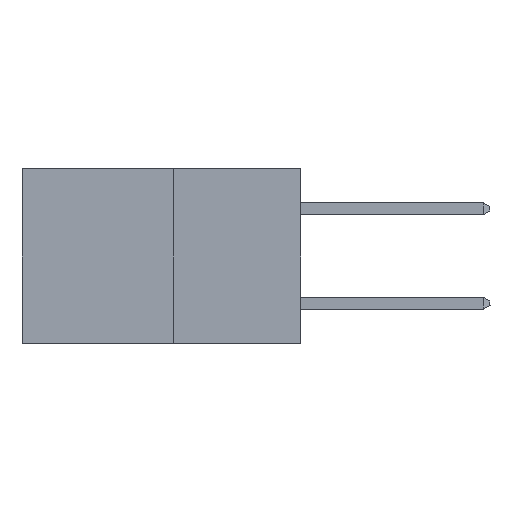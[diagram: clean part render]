
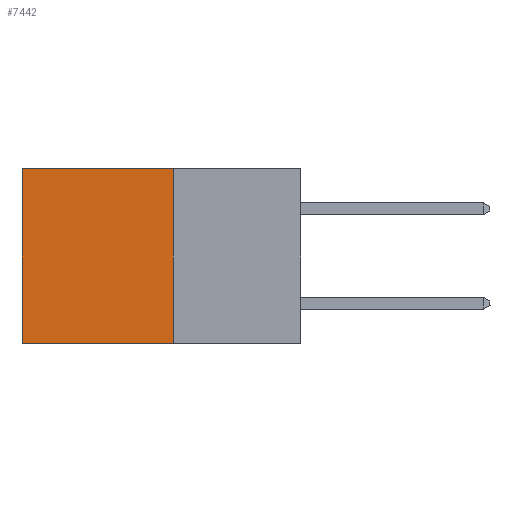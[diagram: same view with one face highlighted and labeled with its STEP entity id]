
A CAD part, left-side view. The second image highlights one B-rep face of the part: STEP entity #7442.
In plain terms, the highlighted planar face has unit normal (-1, 0, 0).
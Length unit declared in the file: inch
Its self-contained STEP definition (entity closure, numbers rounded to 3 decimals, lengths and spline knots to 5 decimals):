
#1515 = EDGE_LOOP ( 'NONE', ( #19555, #17961, #22733, #8371 ) ) ;
#1623 = LINE ( 'NONE', #22899, #10051 ) ;
#2425 = LINE ( 'NONE', #10143, #11977 ) ;
#2489 = VERTEX_POINT ( 'NONE', #14264 ) ;
#5744 = VERTEX_POINT ( 'NONE', #11250 ) ;
#7442 = ADVANCED_FACE ( 'NONE', ( #20026 ), #17059, .F. ) ;
#7711 = EDGE_CURVE ( 'NONE', #5744, #18643, #14528, .T. ) ;
#7771 = DIRECTION ( 'NONE',  ( 0., 0., -1. ) ) ;
#8371 = ORIENTED_EDGE ( 'NONE', *, *, #14161, .T. ) ;
#10039 = DIRECTION ( 'NONE',  ( 1., 0., 0. ) ) ;
#10051 = VECTOR ( 'NONE', #12383, 39.37008 ) ;
#10143 = CARTESIAN_POINT ( 'NONE',  ( 0.277, 0.27, -0.37 ) ) ;
#11250 = CARTESIAN_POINT ( 'NONE',  ( 0.277, 0.27, 0. ) ) ;
#11953 = VERTEX_POINT ( 'NONE', #12221 ) ;
#11977 = VECTOR ( 'NONE', #17158, 39.37008 ) ;
#12046 = CARTESIAN_POINT ( 'NONE',  ( 0.277, 0.27, -0.37 ) ) ;
#12221 = CARTESIAN_POINT ( 'NONE',  ( 0.277, 0.59, 0. ) ) ;
#12383 = DIRECTION ( 'NONE',  ( 0., 1., 0. ) ) ;
#14016 = AXIS2_PLACEMENT_3D ( 'NONE', #20571, #10039, #22344 ) ;
#14161 = EDGE_CURVE ( 'NONE', #5744, #11953, #1623, .T. ) ;
#14262 = CARTESIAN_POINT ( 'NONE',  ( 0.277, 0.27, -0.37 ) ) ;
#14264 = CARTESIAN_POINT ( 'NONE',  ( 0.277, 0.59, -0.37 ) ) ;
#14528 = LINE ( 'NONE', #14262, #18631 ) ;
#16034 = DIRECTION ( 'NONE',  ( 0., 0., -1. ) ) ;
#16589 = CARTESIAN_POINT ( 'NONE',  ( 0.277, 0.59, -0.37 ) ) ;
#17059 = PLANE ( 'NONE',  #14016 ) ;
#17158 = DIRECTION ( 'NONE',  ( 0., 1., 0. ) ) ;
#17363 = EDGE_CURVE ( 'NONE', #18643, #2489, #2425, .T. ) ;
#17867 = VECTOR ( 'NONE', #7771, 39.37008 ) ;
#17961 = ORIENTED_EDGE ( 'NONE', *, *, #17363, .F. ) ;
#18631 = VECTOR ( 'NONE', #16034, 39.37008 ) ;
#18643 = VERTEX_POINT ( 'NONE', #12046 ) ;
#19555 = ORIENTED_EDGE ( 'NONE', *, *, #19784, .T. ) ;
#19784 = EDGE_CURVE ( 'NONE', #11953, #2489, #22558, .T. ) ;
#20026 = FACE_OUTER_BOUND ( 'NONE', #1515, .T. ) ;
#20571 = CARTESIAN_POINT ( 'NONE',  ( 0.277, 0.27, -0.37 ) ) ;
#22344 = DIRECTION ( 'NONE',  ( 0., 0., -1. ) ) ;
#22558 = LINE ( 'NONE', #16589, #17867 ) ;
#22733 = ORIENTED_EDGE ( 'NONE', *, *, #7711, .F. ) ;
#22899 = CARTESIAN_POINT ( 'NONE',  ( 0.277, 0.27, 0. ) ) ;
